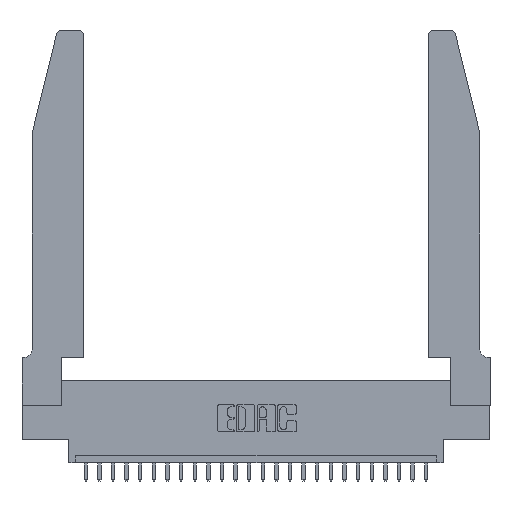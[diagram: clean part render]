
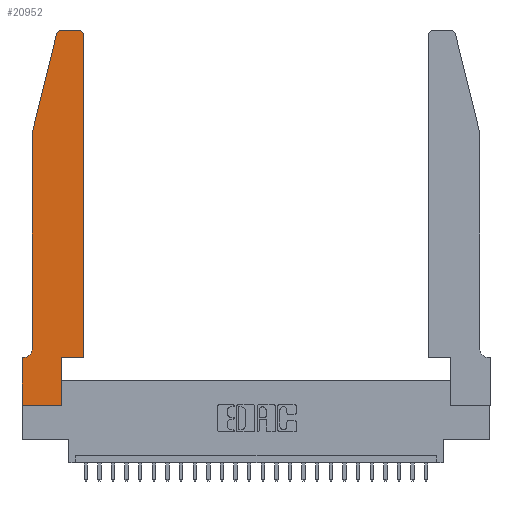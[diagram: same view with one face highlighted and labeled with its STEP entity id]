
A CAD part, top view. The second image highlights one B-rep face of the part: STEP entity #20952.
In plain terms, the highlighted planar face has unit normal (0, 0, 1).
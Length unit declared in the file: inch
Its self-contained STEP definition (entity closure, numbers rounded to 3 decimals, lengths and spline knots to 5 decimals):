
#47 = DIRECTION ( 'NONE',  ( 1., 0., 0. ) ) ;
#224 = CARTESIAN_POINT ( 'NONE',  ( 0.0755, 0.35, 0.37 ) ) ;
#569 = CIRCLE ( 'NONE', #22603, 0.03 ) ;
#714 = CARTESIAN_POINT ( 'NONE',  ( 0.25487, 2.72718, 0.37 ) ) ;
#949 = ORIENTED_EDGE ( 'NONE', *, *, #19535, .T. ) ;
#966 = CARTESIAN_POINT ( 'NONE',  ( 0.4205, 2.75, 0.37 ) ) ;
#1004 = ORIENTED_EDGE ( 'NONE', *, *, #15650, .T. ) ;
#1565 = VERTEX_POINT ( 'NONE', #23008 ) ;
#1566 = DIRECTION ( 'NONE',  ( 0., 0., 1. ) ) ;
#1728 = VECTOR ( 'NONE', #23709, 39.37008 ) ;
#1740 = CARTESIAN_POINT ( 'NONE',  ( 0., 0., 0.37 ) ) ;
#1794 = CARTESIAN_POINT ( 'NONE',  ( 0.4505, 0.35, 0.37 ) ) ;
#1828 = VERTEX_POINT ( 'NONE', #714 ) ;
#1944 = VECTOR ( 'NONE', #16671, 39.37008 ) ;
#2355 = LINE ( 'NONE', #15951, #1728 ) ;
#2372 = DIRECTION ( 'NONE',  ( 0., 0., 1. ) ) ;
#2411 = ORIENTED_EDGE ( 'NONE', *, *, #26034, .T. ) ;
#2628 = CIRCLE ( 'NONE', #2788, 0.07 ) ;
#2788 = AXIS2_PLACEMENT_3D ( 'NONE', #16518, #22588, #4304 ) ;
#3525 = CARTESIAN_POINT ( 'NONE',  ( 0.2605, 2.75, 0.37 ) ) ;
#3538 = VECTOR ( 'NONE', #16640, 39.37008 ) ;
#3596 = VERTEX_POINT ( 'NONE', #20468 ) ;
#4304 = DIRECTION ( 'NONE',  ( -1., 0., 0. ) ) ;
#4494 = VECTOR ( 'NONE', #23187, 39.37008 ) ;
#4996 = CARTESIAN_POINT ( 'NONE',  ( 0., 0.35, 0.37 ) ) ;
#5530 = DIRECTION ( 'NONE',  ( 1., 0., 0. ) ) ;
#5842 = LINE ( 'NONE', #10321, #3538 ) ;
#6243 = ORIENTED_EDGE ( 'NONE', *, *, #21440, .T. ) ;
#6415 = DIRECTION ( 'NONE',  ( 1., 0., 0. ) ) ;
#6475 = EDGE_CURVE ( 'NONE', #19157, #25682, #2355, .T. ) ;
#6852 = CARTESIAN_POINT ( 'NONE',  ( 0.284, 2.72, 0.37 ) ) ;
#6883 = DIRECTION ( 'NONE',  ( 0., 1., 0. ) ) ;
#7192 = LINE ( 'NONE', #1740, #12021 ) ;
#7317 = LINE ( 'NONE', #20366, #26577 ) ;
#7587 = VERTEX_POINT ( 'NONE', #966 ) ;
#7775 = ORIENTED_EDGE ( 'NONE', *, *, #21090, .T. ) ;
#7860 = ORIENTED_EDGE ( 'NONE', *, *, #12981, .T. ) ;
#8386 = FACE_OUTER_BOUND ( 'NONE', #21535, .T. ) ;
#9111 = VECTOR ( 'NONE', #23929, 39.37008 ) ;
#9395 = ORIENTED_EDGE ( 'NONE', *, *, #16150, .T. ) ;
#9781 = EDGE_CURVE ( 'NONE', #1565, #1828, #569, .T. ) ;
#10112 = VERTEX_POINT ( 'NONE', #16237 ) ;
#10321 = CARTESIAN_POINT ( 'NONE',  ( 0., 0., 0.37 ) ) ;
#10595 = VECTOR ( 'NONE', #6415, 39.37008 ) ;
#10711 = VERTEX_POINT ( 'NONE', #4996 ) ;
#11372 = AXIS2_PLACEMENT_3D ( 'NONE', #11939, #1566, #5530 ) ;
#11553 = ORIENTED_EDGE ( 'NONE', *, *, #17897, .T. ) ;
#11893 = LINE ( 'NONE', #24000, #10595 ) ;
#11939 = CARTESIAN_POINT ( 'NONE',  ( 0.4205, 2.72, 0.37 ) ) ;
#11981 = ORIENTED_EDGE ( 'NONE', *, *, #26504, .T. ) ;
#12021 = VECTOR ( 'NONE', #15847, 39.37008 ) ;
#12374 = VERTEX_POINT ( 'NONE', #16836 ) ;
#12628 = CARTESIAN_POINT ( 'NONE',  ( 0.4505, 2.72, 0.37 ) ) ;
#12753 = CARTESIAN_POINT ( 'NONE',  ( 0.0755, 2., 0.37 ) ) ;
#12925 = LINE ( 'NONE', #224, #1944 ) ;
#12970 = DIRECTION ( 'NONE',  ( 0., 0., 1. ) ) ;
#12981 = EDGE_CURVE ( 'NONE', #15499, #3596, #23144, .T. ) ;
#14678 = PLANE ( 'NONE',  #22493 ) ;
#14988 = DIRECTION ( 'NONE',  ( 1., 0., 0. ) ) ;
#15499 = VERTEX_POINT ( 'NONE', #25110 ) ;
#15650 = EDGE_CURVE ( 'NONE', #12374, #15499, #7192, .T. ) ;
#15847 = DIRECTION ( 'NONE',  ( 1., 0., 0. ) ) ;
#15951 = CARTESIAN_POINT ( 'NONE',  ( 0.4505, 0.35, 0.37 ) ) ;
#16150 = EDGE_CURVE ( 'NONE', #10112, #26425, #2628, .T. ) ;
#16237 = CARTESIAN_POINT ( 'NONE',  ( 0.0755, 0.42, 0.37 ) ) ;
#16518 = CARTESIAN_POINT ( 'NONE',  ( 0.0055, 0.42, 0.37 ) ) ;
#16601 = CARTESIAN_POINT ( 'NONE',  ( 0.0055, 0.35, 0.37 ) ) ;
#16640 = DIRECTION ( 'NONE',  ( 0., -1., 0. ) ) ;
#16671 = DIRECTION ( 'NONE',  ( -1., 0., 0. ) ) ;
#16723 = ORIENTED_EDGE ( 'NONE', *, *, #16748, .T. ) ;
#16748 = EDGE_CURVE ( 'NONE', #26425, #10711, #12925, .T. ) ;
#16836 = CARTESIAN_POINT ( 'NONE',  ( 0., 0., 0.37 ) ) ;
#17171 = CARTESIAN_POINT ( 'NONE',  ( 0.2865, 0.35, 0.37 ) ) ;
#17189 = VERTEX_POINT ( 'NONE', #25976 ) ;
#17357 = LINE ( 'NONE', #12753, #4494 ) ;
#17395 = LINE ( 'NONE', #3525, #9111 ) ;
#17721 = VECTOR ( 'NONE', #6883, 39.37008 ) ;
#17897 = EDGE_CURVE ( 'NONE', #3596, #19157, #11893, .T. ) ;
#18268 = ORIENTED_EDGE ( 'NONE', *, *, #9781, .T. ) ;
#19157 = VERTEX_POINT ( 'NONE', #1794 ) ;
#19250 = ORIENTED_EDGE ( 'NONE', *, *, #6475, .T. ) ;
#19535 = EDGE_CURVE ( 'NONE', #25682, #7587, #21741, .T. ) ;
#20366 = CARTESIAN_POINT ( 'NONE',  ( 0.0755, 2., 0.37 ) ) ;
#20468 = CARTESIAN_POINT ( 'NONE',  ( 0.2865, 0.35, 0.37 ) ) ;
#20952 = ADVANCED_FACE ( 'NONE', ( #8386 ), #14678, .T. ) ;
#21090 = EDGE_CURVE ( 'NONE', #17189, #10112, #17357, .T. ) ;
#21440 = EDGE_CURVE ( 'NONE', #10711, #12374, #5842, .T. ) ;
#21535 = EDGE_LOOP ( 'NONE', ( #2411, #18268, #11981, #7775, #9395, #16723, #6243, #1004, #7860, #11553, #19250, #949 ) ) ;
#21741 = CIRCLE ( 'NONE', #11372, 0.03 ) ;
#22493 = AXIS2_PLACEMENT_3D ( 'NONE', #22554, #2372, #47 ) ;
#22554 = CARTESIAN_POINT ( 'NONE',  ( 0., 0.35, 0.37 ) ) ;
#22588 = DIRECTION ( 'NONE',  ( 0., 0., -1. ) ) ;
#22603 = AXIS2_PLACEMENT_3D ( 'NONE', #6852, #12970, #14988 ) ;
#23008 = CARTESIAN_POINT ( 'NONE',  ( 0.284, 2.75, 0.37 ) ) ;
#23144 = LINE ( 'NONE', #17171, #17721 ) ;
#23187 = DIRECTION ( 'NONE',  ( 0., -1., 0. ) ) ;
#23709 = DIRECTION ( 'NONE',  ( 0., 1., 0. ) ) ;
#23929 = DIRECTION ( 'NONE',  ( -1., 0., 0. ) ) ;
#24000 = CARTESIAN_POINT ( 'NONE',  ( 0.4505, 0.35, 0.37 ) ) ;
#24008 = DIRECTION ( 'NONE',  ( -0.239, -0.971, 0. ) ) ;
#25110 = CARTESIAN_POINT ( 'NONE',  ( 0.2865, 0., 0.37 ) ) ;
#25682 = VERTEX_POINT ( 'NONE', #12628 ) ;
#25976 = CARTESIAN_POINT ( 'NONE',  ( 0.0755, 2., 0.37 ) ) ;
#26034 = EDGE_CURVE ( 'NONE', #7587, #1565, #17395, .T. ) ;
#26425 = VERTEX_POINT ( 'NONE', #16601 ) ;
#26504 = EDGE_CURVE ( 'NONE', #1828, #17189, #7317, .T. ) ;
#26577 = VECTOR ( 'NONE', #24008, 39.37008 ) ;
